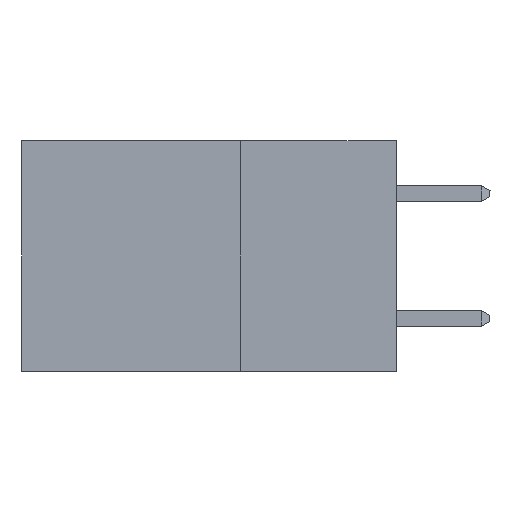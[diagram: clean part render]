
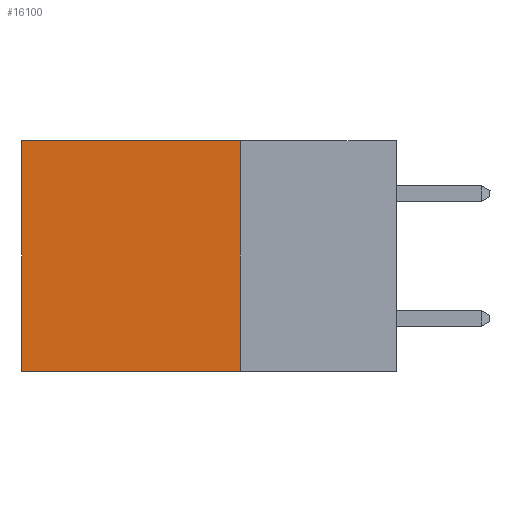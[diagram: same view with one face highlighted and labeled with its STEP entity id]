
A CAD part, left-side view. The second image highlights one B-rep face of the part: STEP entity #16100.
In plain terms, the highlighted planar face has unit normal (-1, 0, 0).
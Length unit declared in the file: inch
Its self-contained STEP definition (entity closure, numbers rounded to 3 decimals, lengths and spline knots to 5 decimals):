
#12 = ORIENTED_EDGE ( 'NONE', *, *, #13383, .T. ) ;
#253 = LINE ( 'NONE', #2895, #10755 ) ;
#270 = VECTOR ( 'NONE', #7174, 39.37008 ) ;
#683 = CARTESIAN_POINT ( 'NONE',  ( 0.298, 0.6, 0. ) ) ;
#926 = VECTOR ( 'NONE', #9141, 39.37008 ) ;
#2722 = CARTESIAN_POINT ( 'NONE',  ( 0.298, 0.25, 0. ) ) ;
#2895 = CARTESIAN_POINT ( 'NONE',  ( 0.298, 0.25, 0. ) ) ;
#3211 = EDGE_LOOP ( 'NONE', ( #12, #10261, #13068, #17550 ) ) ;
#3531 = CARTESIAN_POINT ( 'NONE',  ( 0.298, 0.6, -0.37 ) ) ;
#3551 = CARTESIAN_POINT ( 'NONE',  ( 0.298, 0.25, -0.37 ) ) ;
#4064 = DIRECTION ( 'NONE',  ( 0., 0., -1. ) ) ;
#4370 = EDGE_CURVE ( 'NONE', #12746, #13422, #14918, .T. ) ;
#4766 = LINE ( 'NONE', #683, #12579 ) ;
#4969 = VERTEX_POINT ( 'NONE', #10128 ) ;
#7174 = DIRECTION ( 'NONE',  ( 0., 1., 0. ) ) ;
#7734 = CARTESIAN_POINT ( 'NONE',  ( 0.298, 0.25, 0. ) ) ;
#8771 = AXIS2_PLACEMENT_3D ( 'NONE', #2722, #12330, #4064 ) ;
#8872 = DIRECTION ( 'NONE',  ( 0., 0., -1. ) ) ;
#9141 = DIRECTION ( 'NONE',  ( 0., 1., 0. ) ) ;
#10005 = VERTEX_POINT ( 'NONE', #12537 ) ;
#10128 = CARTESIAN_POINT ( 'NONE',  ( 0.298, 0.25, 0. ) ) ;
#10261 = ORIENTED_EDGE ( 'NONE', *, *, #4370, .F. ) ;
#10755 = VECTOR ( 'NONE', #11052, 39.37008 ) ;
#10882 = PLANE ( 'NONE',  #8771 ) ;
#11052 = DIRECTION ( 'NONE',  ( 0., 0., -1. ) ) ;
#12330 = DIRECTION ( 'NONE',  ( 1., 0., 0. ) ) ;
#12537 = CARTESIAN_POINT ( 'NONE',  ( 0.298, 0.6, 0. ) ) ;
#12579 = VECTOR ( 'NONE', #8872, 39.37008 ) ;
#12746 = VERTEX_POINT ( 'NONE', #3551 ) ;
#13068 = ORIENTED_EDGE ( 'NONE', *, *, #14317, .F. ) ;
#13383 = EDGE_CURVE ( 'NONE', #10005, #13422, #4766, .T. ) ;
#13402 = FACE_OUTER_BOUND ( 'NONE', #3211, .T. ) ;
#13422 = VERTEX_POINT ( 'NONE', #3531 ) ;
#14012 = EDGE_CURVE ( 'NONE', #4969, #10005, #15543, .T. ) ;
#14317 = EDGE_CURVE ( 'NONE', #4969, #12746, #253, .T. ) ;
#14918 = LINE ( 'NONE', #17594, #270 ) ;
#15543 = LINE ( 'NONE', #7734, #926 ) ;
#16100 = ADVANCED_FACE ( 'NONE', ( #13402 ), #10882, .F. ) ;
#17550 = ORIENTED_EDGE ( 'NONE', *, *, #14012, .T. ) ;
#17594 = CARTESIAN_POINT ( 'NONE',  ( 0.298, 0.25, -0.37 ) ) ;
